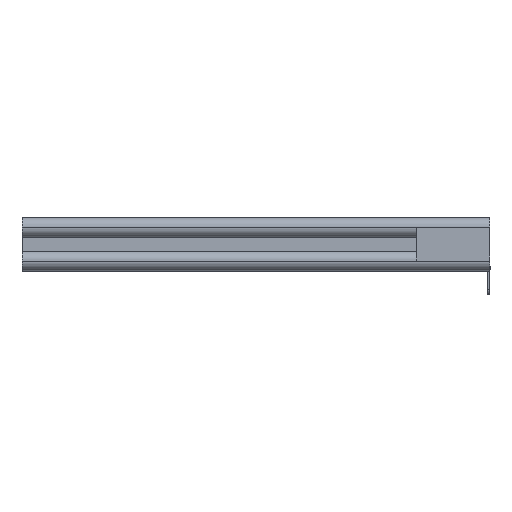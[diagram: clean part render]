
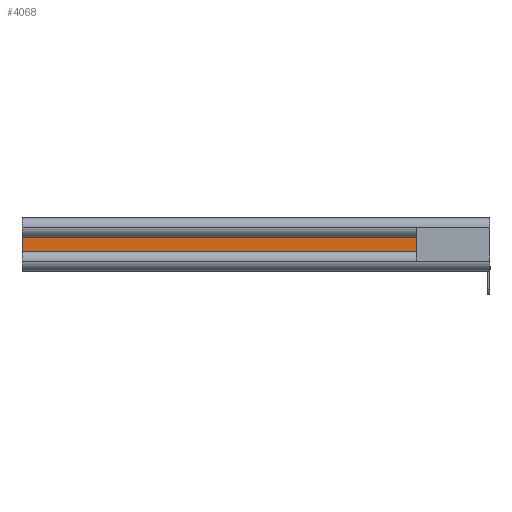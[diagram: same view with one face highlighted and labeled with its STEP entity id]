
A CAD part, left-side view. The second image highlights one B-rep face of the part: STEP entity #4068.
In plain terms, the highlighted planar face has unit normal (-1, 0, 0).
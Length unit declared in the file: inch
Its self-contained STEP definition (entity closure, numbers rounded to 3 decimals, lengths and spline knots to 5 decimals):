
#138 = CARTESIAN_POINT ( 'NONE',  ( 0.044, 0.37012, -0.0465 ) ) ;
#461 = LINE ( 'NONE', #10956, #4961 ) ;
#934 = CARTESIAN_POINT ( 'NONE',  ( 0.044, 0.473, 0.0465 ) ) ;
#2281 = CARTESIAN_POINT ( 'NONE',  ( 0.044, 0.473, -0.0465 ) ) ;
#4068 = ADVANCED_FACE ( 'NONE', ( #13867 ), #15090, .F. ) ;
#4648 = AXIS2_PLACEMENT_3D ( 'NONE', #138, #20534, #9671 ) ;
#4757 = VERTEX_POINT ( 'NONE', #19249 ) ;
#4961 = VECTOR ( 'NONE', #5422, 39.37008 ) ;
#5406 = VERTEX_POINT ( 'NONE', #22758 ) ;
#5422 = DIRECTION ( 'NONE',  ( 0., 1., 0. ) ) ;
#5671 = EDGE_CURVE ( 'NONE', #8007, #4757, #7441, .T. ) ;
#7141 = DIRECTION ( 'NONE',  ( 0., 1., 0. ) ) ;
#7441 = LINE ( 'NONE', #16277, #20830 ) ;
#7610 = LINE ( 'NONE', #18120, #11957 ) ;
#8007 = VERTEX_POINT ( 'NONE', #934 ) ;
#8250 = VECTOR ( 'NONE', #14986, 39.37008 ) ;
#9671 = DIRECTION ( 'NONE',  ( 0., 0., -1. ) ) ;
#9690 = EDGE_CURVE ( 'NONE', #8007, #14946, #23309, .T. ) ;
#10836 = EDGE_CURVE ( 'NONE', #14946, #5406, #461, .T. ) ;
#10956 = CARTESIAN_POINT ( 'NONE',  ( 0.044, 0.37012, -0.0465 ) ) ;
#11957 = VECTOR ( 'NONE', #23557, 39.37008 ) ;
#12133 = EDGE_LOOP ( 'NONE', ( #14990, #17743, #22383, #12256 ) ) ;
#12256 = ORIENTED_EDGE ( 'NONE', *, *, #9690, .F. ) ;
#13168 = CARTESIAN_POINT ( 'NONE',  ( 0.044, 0.473, -0.0465 ) ) ;
#13867 = FACE_OUTER_BOUND ( 'NONE', #12133, .T. ) ;
#14946 = VERTEX_POINT ( 'NONE', #2281 ) ;
#14986 = DIRECTION ( 'NONE',  ( 0., 0., -1. ) ) ;
#14990 = ORIENTED_EDGE ( 'NONE', *, *, #5671, .T. ) ;
#15090 = PLANE ( 'NONE',  #4648 ) ;
#16277 = CARTESIAN_POINT ( 'NONE',  ( 0.044, 0.37012, 0.0465 ) ) ;
#17743 = ORIENTED_EDGE ( 'NONE', *, *, #20790, .T. ) ;
#18120 = CARTESIAN_POINT ( 'NONE',  ( 0.044, 3., -0.0465 ) ) ;
#19249 = CARTESIAN_POINT ( 'NONE',  ( 0.044, 3., 0.0465 ) ) ;
#20534 = DIRECTION ( 'NONE',  ( 1., 0., 0. ) ) ;
#20790 = EDGE_CURVE ( 'NONE', #4757, #5406, #7610, .T. ) ;
#20830 = VECTOR ( 'NONE', #7141, 39.37008 ) ;
#22383 = ORIENTED_EDGE ( 'NONE', *, *, #10836, .F. ) ;
#22758 = CARTESIAN_POINT ( 'NONE',  ( 0.044, 3., -0.0465 ) ) ;
#23309 = LINE ( 'NONE', #13168, #8250 ) ;
#23557 = DIRECTION ( 'NONE',  ( 0., 0., -1. ) ) ;
